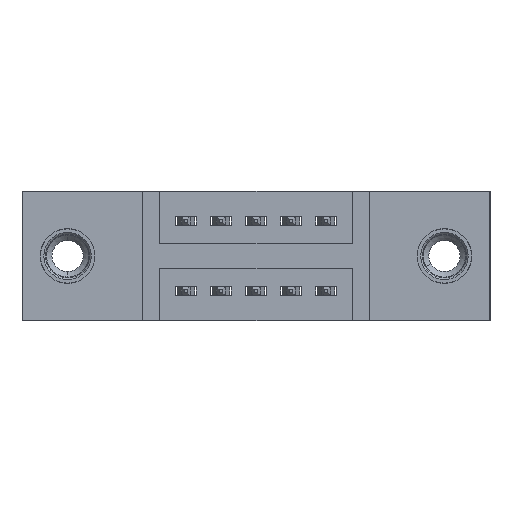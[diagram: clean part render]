
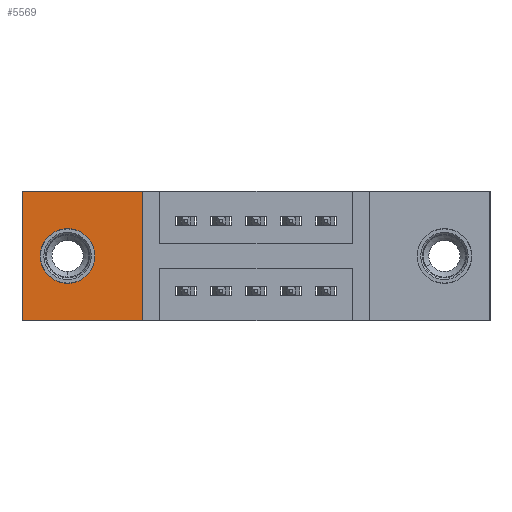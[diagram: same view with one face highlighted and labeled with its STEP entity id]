
A CAD part, front view. The second image highlights one B-rep face of the part: STEP entity #5569.
In plain terms, the highlighted planar face has unit normal (0, -1, 0).
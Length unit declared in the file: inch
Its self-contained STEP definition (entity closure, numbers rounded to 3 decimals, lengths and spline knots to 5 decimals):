
#191 = DIRECTION ( 'NONE',  ( 0., -1., 0. ) ) ;
#505 = DIRECTION ( 'NONE',  ( 0., -1., 0. ) ) ;
#863 = CARTESIAN_POINT ( 'NONE',  ( 0., 0.17, 0. ) ) ;
#1239 = LINE ( 'NONE', #2983, #5617 ) ;
#1281 = DIRECTION ( 'NONE',  ( 0., 0., 1. ) ) ;
#1290 = EDGE_LOOP ( 'NONE', ( #8622, #3358 ) ) ;
#1524 = VERTEX_POINT ( 'NONE', #863 ) ;
#1530 = EDGE_CURVE ( 'NONE', #10241, #1767, #4498, .T. ) ;
#1767 = VERTEX_POINT ( 'NONE', #5151 ) ;
#1881 = CARTESIAN_POINT ( 'NONE',  ( 0.13, 0.17, -0.263 ) ) ;
#1953 = VECTOR ( 'NONE', #1281, 39.37008 ) ;
#2083 = CARTESIAN_POINT ( 'NONE',  ( 0., 0.17, -0.37 ) ) ;
#2285 = ORIENTED_EDGE ( 'NONE', *, *, #6207, .T. ) ;
#2459 = VECTOR ( 'NONE', #8008, 39.37008 ) ;
#2595 = CARTESIAN_POINT ( 'NONE',  ( 0.3425, 0.17, -0.37 ) ) ;
#2599 = CARTESIAN_POINT ( 'NONE',  ( 0., 0.17, 0. ) ) ;
#2905 = CARTESIAN_POINT ( 'NONE',  ( 0.3425, 0.17, 0. ) ) ;
#2959 = CARTESIAN_POINT ( 'NONE',  ( 0., 0.17, -0.37 ) ) ;
#2983 = CARTESIAN_POINT ( 'NONE',  ( 0., 0.17, 0. ) ) ;
#3123 = AXIS2_PLACEMENT_3D ( 'NONE', #4583, #5084, #6885 ) ;
#3205 = ORIENTED_EDGE ( 'NONE', *, *, #7643, .T. ) ;
#3238 = LINE ( 'NONE', #2083, #7292 ) ;
#3358 = ORIENTED_EDGE ( 'NONE', *, *, #1530, .F. ) ;
#3809 = ORIENTED_EDGE ( 'NONE', *, *, #6080, .T. ) ;
#4079 = FACE_OUTER_BOUND ( 'NONE', #7769, .T. ) ;
#4270 = EDGE_CURVE ( 'NONE', #1767, #10241, #7982, .T. ) ;
#4285 = VERTEX_POINT ( 'NONE', #2905 ) ;
#4336 = FACE_BOUND ( 'NONE', #1290, .T. ) ;
#4430 = LINE ( 'NONE', #9095, #1953 ) ;
#4498 = CIRCLE ( 'NONE', #3123, 0.078 ) ;
#4583 = CARTESIAN_POINT ( 'NONE',  ( 0.13, 0.17, -0.185 ) ) ;
#4717 = AXIS2_PLACEMENT_3D ( 'NONE', #5263, #191, #6036 ) ;
#4728 = CARTESIAN_POINT ( 'NONE',  ( 0., 0.17, -0.37 ) ) ;
#4929 = AXIS2_PLACEMENT_3D ( 'NONE', #4728, #505, #6278 ) ;
#5084 = DIRECTION ( 'NONE',  ( 0., -1., 0. ) ) ;
#5151 = CARTESIAN_POINT ( 'NONE',  ( 0.13, 0.17, -0.107 ) ) ;
#5263 = CARTESIAN_POINT ( 'NONE',  ( 0.13, 0.17, -0.185 ) ) ;
#5569 = ADVANCED_FACE ( 'NONE', ( #4336, #4079 ), #9208, .T. ) ;
#5617 = VECTOR ( 'NONE', #8315, 39.37008 ) ;
#6036 = DIRECTION ( 'NONE',  ( 0., 0., -1. ) ) ;
#6080 = EDGE_CURVE ( 'NONE', #4285, #1524, #1239, .T. ) ;
#6207 = EDGE_CURVE ( 'NONE', #10125, #4285, #4430, .T. ) ;
#6278 = DIRECTION ( 'NONE',  ( 0., 0., -1. ) ) ;
#6418 = LINE ( 'NONE', #2599, #2459 ) ;
#6802 = DIRECTION ( 'NONE',  ( 1., 0., 0. ) ) ;
#6885 = DIRECTION ( 'NONE',  ( 0., 0., -1. ) ) ;
#7292 = VECTOR ( 'NONE', #6802, 39.37008 ) ;
#7351 = ORIENTED_EDGE ( 'NONE', *, *, #9224, .T. ) ;
#7643 = EDGE_CURVE ( 'NONE', #1524, #8430, #6418, .T. ) ;
#7769 = EDGE_LOOP ( 'NONE', ( #3205, #7351, #2285, #3809 ) ) ;
#7982 = CIRCLE ( 'NONE', #4717, 0.078 ) ;
#8008 = DIRECTION ( 'NONE',  ( 0., 0., -1. ) ) ;
#8315 = DIRECTION ( 'NONE',  ( -1., 0., 0. ) ) ;
#8430 = VERTEX_POINT ( 'NONE', #2959 ) ;
#8622 = ORIENTED_EDGE ( 'NONE', *, *, #4270, .F. ) ;
#9095 = CARTESIAN_POINT ( 'NONE',  ( 0.3425, 0.17, 0. ) ) ;
#9208 = PLANE ( 'NONE',  #4929 ) ;
#9224 = EDGE_CURVE ( 'NONE', #8430, #10125, #3238, .T. ) ;
#10125 = VERTEX_POINT ( 'NONE', #2595 ) ;
#10241 = VERTEX_POINT ( 'NONE', #1881 ) ;
